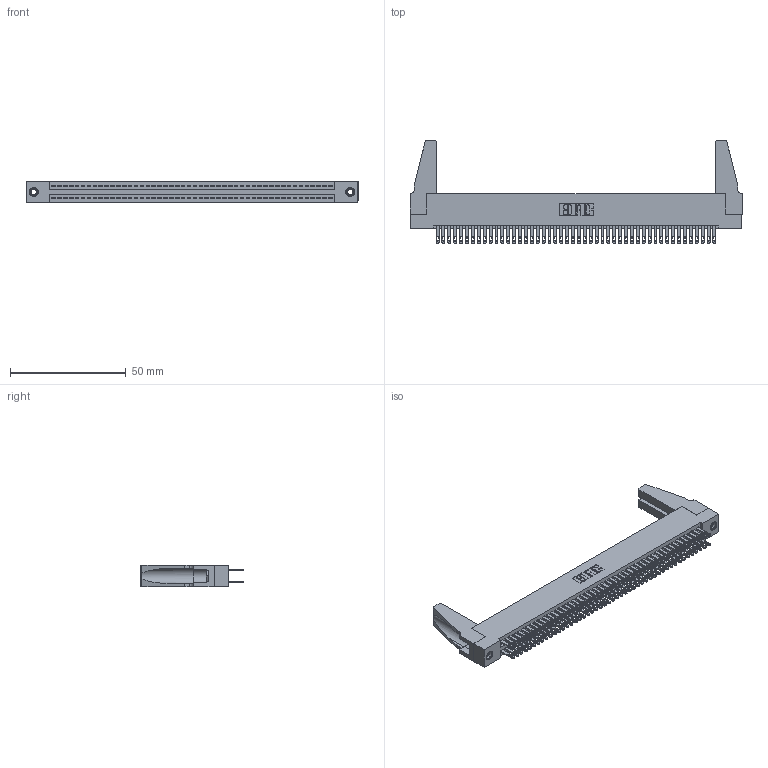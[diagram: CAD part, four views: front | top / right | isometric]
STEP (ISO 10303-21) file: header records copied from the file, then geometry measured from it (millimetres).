
FILE_DESCRIPTION (( 'STEP AP203' ), '1' );
FILE_NAME ('345-096-500-288.STEP', '2019-11-02T06:31:21', ( '' ), ( '' ), 'SwSTEP 2.0', 'SolidWorks 2016', '' );
FILE_SCHEMA (( 'CONFIG_CONTROL_DESIGN' ));
Length unit declared in the file: inch
Products named in the file (5): 345-096-500-288; 345-292-001_345-293-100; 345 Part_Flush Mounting Lugs - 0.156 Dia-TH; 345-220-078_345-220-088; 345-250-001_345-250-001-102
Assembly tree (101 placements, depth 2):
  345-096-500-288
    345 Part_Flush Mounting Lugs - 0.156 Dia-TH
    345-292-001_345-293-100  x96
    345-250-001_345-250-001-102  x2
    345-220-078_345-220-088  x2
Bounding box: 143.15 x 44.37 x 9.4 mm (x, y, z)
Volume: 17507.7 mm3; surface area: 25289.1 mm2
Topology: 101 solids, 101 shells, 4666 faces, 14191 edges, 9450 vertices
Faces by surface type: plane 2744, cylinder 1906, cone 12, torus 4
Entity records: 38932 total; most frequent: CARTESIAN_POINT 6514, ORIENTED_EDGE 6408, DIRECTION 5744, EDGE_CURVE 3204, VECTOR 2834, LINE 2834, VERTEX_POINT 2130, AXIS2_PLACEMENT_3D 1455
